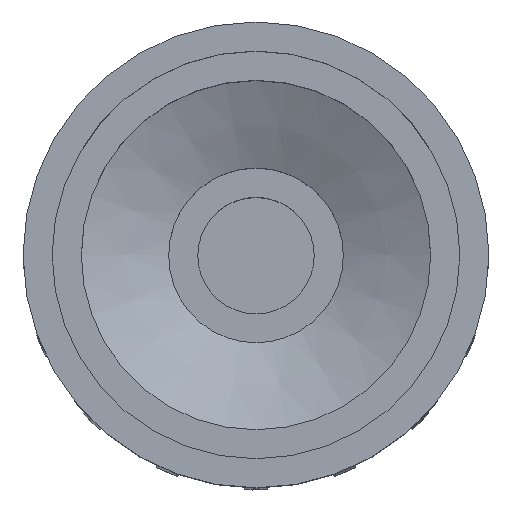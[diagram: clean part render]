
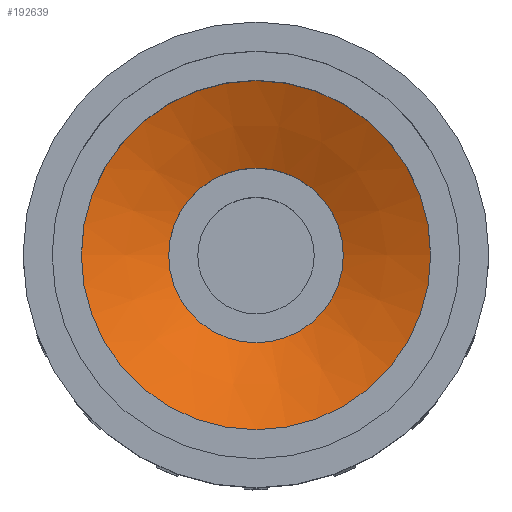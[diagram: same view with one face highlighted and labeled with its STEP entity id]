
A CAD part, top view. The second image highlights one B-rep face of the part: STEP entity #192639.
In plain terms, the highlighted conical face has half-angle 66.038 degrees and reference radius 9.525 mm.
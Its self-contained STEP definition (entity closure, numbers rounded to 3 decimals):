
#192573 = CYLINDRICAL_SURFACE('',#192574,19.05);
#192574 = AXIS2_PLACEMENT_3D('',#192575,#192576,#192577);
#192575 = CARTESIAN_POINT('',(0.,0.,113.285));
#192576 = DIRECTION('',(0.,0.,1.));
#192577 = DIRECTION('',(-1.,0.,0.));
#192590 = VERTEX_POINT('',#192591);
#192591 = CARTESIAN_POINT('',(-19.05,0.,113.285));
#192612 = EDGE_CURVE('',#192590,#192590,#192613,.T.);
#192613 = SURFACE_CURVE('',#192614,(#192619,#192626),.PCURVE_S1.);
#192614 = CIRCLE('',#192615,19.05);
#192615 = AXIS2_PLACEMENT_3D('',#192616,#192617,#192618);
#192616 = CARTESIAN_POINT('',(0.,0.,113.285));
#192617 = DIRECTION('',(0.,0.,1.));
#192618 = DIRECTION('',(-1.,0.,0.));
#192619 = PCURVE('',#192573,#192620);
#192620 = DEFINITIONAL_REPRESENTATION('',(#192621),#192625);
#192621 = LINE('',#192622,#192623);
#192622 = CARTESIAN_POINT('',(0.,0.));
#192623 = VECTOR('',#192624,1.);
#192624 = DIRECTION('',(1.,0.));
#192625 = ( GEOMETRIC_REPRESENTATION_CONTEXT(2) 
PARAMETRIC_REPRESENTATION_CONTEXT() REPRESENTATION_CONTEXT('2D SPACE',''
  ) );
#192626 = PCURVE('',#192627,#192632);
#192627 = CONICAL_SURFACE('',#192628,9.525,1.153);
#192628 = AXIS2_PLACEMENT_3D('',#192629,#192630,#192631);
#192629 = CARTESIAN_POINT('',(0.,0.,109.051));
#192630 = DIRECTION('',(0.,0.,1.));
#192631 = DIRECTION('',(-1.,0.,0.));
#192632 = DEFINITIONAL_REPRESENTATION('',(#192633),#192637);
#192633 = LINE('',#192634,#192635);
#192634 = CARTESIAN_POINT('',(0.,4.233));
#192635 = VECTOR('',#192636,1.);
#192636 = DIRECTION('',(1.,0.));
#192637 = ( GEOMETRIC_REPRESENTATION_CONTEXT(2) 
PARAMETRIC_REPRESENTATION_CONTEXT() REPRESENTATION_CONTEXT('2D SPACE',''
  ) );
#192639 = ADVANCED_FACE('',(#192640),#192627,.F.);
#192640 = FACE_BOUND('',#192641,.F.);
#192641 = EDGE_LOOP('',(#192642,#192643,#192666,#192693));
#192642 = ORIENTED_EDGE('',*,*,#192612,.F.);
#192643 = ORIENTED_EDGE('',*,*,#192644,.F.);
#192644 = EDGE_CURVE('',#192645,#192590,#192647,.T.);
#192645 = VERTEX_POINT('',#192646);
#192646 = CARTESIAN_POINT('',(-9.525,0.,109.051));
#192647 = SEAM_CURVE('',#192648,(#192652,#192659),.PCURVE_S1.);
#192648 = LINE('',#192649,#192650);
#192649 = CARTESIAN_POINT('',(-9.525,0.,109.051));
#192650 = VECTOR('',#192651,1.);
#192651 = DIRECTION('',(-0.914,0.,
    0.406));
#192652 = PCURVE('',#192627,#192653);
#192653 = DEFINITIONAL_REPRESENTATION('',(#192654),#192658);
#192654 = LINE('',#192655,#192656);
#192655 = CARTESIAN_POINT('',(0.,0.));
#192656 = VECTOR('',#192657,1.);
#192657 = DIRECTION('',(0.,1.));
#192658 = ( GEOMETRIC_REPRESENTATION_CONTEXT(2) 
PARAMETRIC_REPRESENTATION_CONTEXT() REPRESENTATION_CONTEXT('2D SPACE',''
  ) );
#192659 = PCURVE('',#192627,#192660);
#192660 = DEFINITIONAL_REPRESENTATION('',(#192661),#192665);
#192661 = LINE('',#192662,#192663);
#192662 = CARTESIAN_POINT('',(6.283,0.));
#192663 = VECTOR('',#192664,1.);
#192664 = DIRECTION('',(0.,1.));
#192665 = ( GEOMETRIC_REPRESENTATION_CONTEXT(2) 
PARAMETRIC_REPRESENTATION_CONTEXT() REPRESENTATION_CONTEXT('2D SPACE',''
  ) );
#192666 = ORIENTED_EDGE('',*,*,#192667,.T.);
#192667 = EDGE_CURVE('',#192645,#192645,#192668,.T.);
#192668 = SURFACE_CURVE('',#192669,(#192674,#192681),.PCURVE_S1.);
#192669 = CIRCLE('',#192670,9.525);
#192670 = AXIS2_PLACEMENT_3D('',#192671,#192672,#192673);
#192671 = CARTESIAN_POINT('',(0.,0.,109.051));
#192672 = DIRECTION('',(0.,0.,1.));
#192673 = DIRECTION('',(-1.,0.,0.));
#192674 = PCURVE('',#192627,#192675);
#192675 = DEFINITIONAL_REPRESENTATION('',(#192676),#192680);
#192676 = LINE('',#192677,#192678);
#192677 = CARTESIAN_POINT('',(0.,0.));
#192678 = VECTOR('',#192679,1.);
#192679 = DIRECTION('',(1.,0.));
#192680 = ( GEOMETRIC_REPRESENTATION_CONTEXT(2) 
PARAMETRIC_REPRESENTATION_CONTEXT() REPRESENTATION_CONTEXT('2D SPACE',''
  ) );
#192681 = PCURVE('',#192682,#192687);
#192682 = CYLINDRICAL_SURFACE('',#192683,9.525);
#192683 = AXIS2_PLACEMENT_3D('',#192684,#192685,#192686);
#192684 = CARTESIAN_POINT('',(0.,0.,96.351));
#192685 = DIRECTION('',(0.,0.,1.));
#192686 = DIRECTION('',(-1.,0.,0.));
#192687 = DEFINITIONAL_REPRESENTATION('',(#192688),#192692);
#192688 = LINE('',#192689,#192690);
#192689 = CARTESIAN_POINT('',(0.,12.7));
#192690 = VECTOR('',#192691,1.);
#192691 = DIRECTION('',(1.,0.));
#192692 = ( GEOMETRIC_REPRESENTATION_CONTEXT(2) 
PARAMETRIC_REPRESENTATION_CONTEXT() REPRESENTATION_CONTEXT('2D SPACE',''
  ) );
#192693 = ORIENTED_EDGE('',*,*,#192644,.T.);
